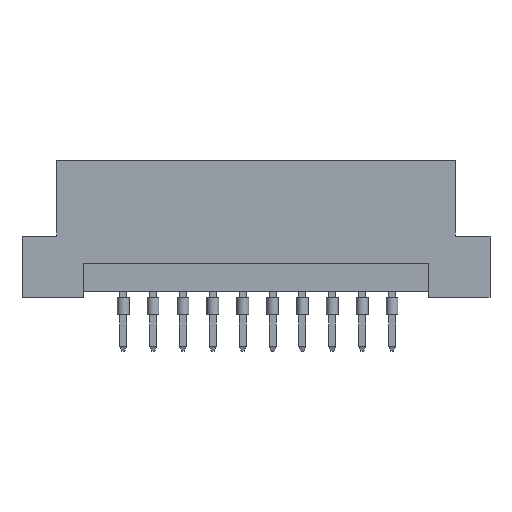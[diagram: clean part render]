
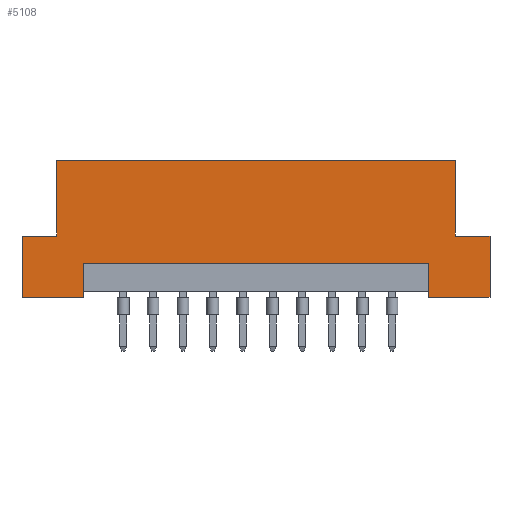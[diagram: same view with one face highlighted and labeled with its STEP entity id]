
A CAD part, front view. The second image highlights one B-rep face of the part: STEP entity #5108.
In plain terms, the highlighted planar face has unit normal (0, -1, 0).
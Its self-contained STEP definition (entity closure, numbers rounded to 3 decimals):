
#150 = CARTESIAN_POINT ( 'NONE',  ( 19.9, 0., 5.2 ) ) ;
#184 = DIRECTION ( 'NONE',  ( 0., 0., -1. ) ) ;
#199 = VECTOR ( 'NONE', #1365, 1000. ) ;
#215 = VERTEX_POINT ( 'NONE', #4006 ) ;
#225 = DIRECTION ( 'NONE',  ( 0., 0., 1. ) ) ;
#230 = LINE ( 'NONE', #5498, #4510 ) ;
#260 = DIRECTION ( 'NONE',  ( -1., 0., 0. ) ) ;
#274 = ORIENTED_EDGE ( 'NONE', *, *, #7486, .F. ) ;
#414 = VECTOR ( 'NONE', #1257, 1000. ) ;
#516 = ORIENTED_EDGE ( 'NONE', *, *, #4968, .F. ) ;
#571 = CARTESIAN_POINT ( 'NONE',  ( -19.9, 0., 5.2 ) ) ;
#603 = AXIS2_PLACEMENT_3D ( 'NONE', #806, #7228, #225 ) ;
#608 = LINE ( 'NONE', #571, #4751 ) ;
#670 = CARTESIAN_POINT ( 'NONE',  ( 16.94, 0., 5.2 ) ) ;
#682 = DIRECTION ( 'NONE',  ( 0., 0., 1. ) ) ;
#714 = DIRECTION ( 'NONE',  ( 0., 0., 1. ) ) ;
#747 = VECTOR ( 'NONE', #714, 1000. ) ;
#806 = CARTESIAN_POINT ( 'NONE',  ( -19.9, 0., 11.6 ) ) ;
#909 = EDGE_CURVE ( 'NONE', #4019, #6713, #3039, .T. ) ;
#1257 = DIRECTION ( 'NONE',  ( 1., 0., 0. ) ) ;
#1327 = CARTESIAN_POINT ( 'NONE',  ( -19.9, 0., 0. ) ) ;
#1365 = DIRECTION ( 'NONE',  ( 1., 0., 0. ) ) ;
#1489 = DIRECTION ( 'NONE',  ( 0., 0., -1. ) ) ;
#1496 = VERTEX_POINT ( 'NONE', #6316 ) ;
#1533 = CARTESIAN_POINT ( 'NONE',  ( 19.9, 0., 0. ) ) ;
#1563 = EDGE_CURVE ( 'NONE', #215, #4696, #6860, .T. ) ;
#1729 = CARTESIAN_POINT ( 'NONE',  ( -19.9, 0., 5.2 ) ) ;
#1744 = ORIENTED_EDGE ( 'NONE', *, *, #5093, .T. ) ;
#1761 = VERTEX_POINT ( 'NONE', #5969 ) ;
#1875 = CARTESIAN_POINT ( 'NONE',  ( 19.9, 0., 0. ) ) ;
#1886 = VECTOR ( 'NONE', #2543, 1000. ) ;
#1890 = VECTOR ( 'NONE', #5689, 1000. ) ;
#2126 = ORIENTED_EDGE ( 'NONE', *, *, #2799, .F. ) ;
#2294 = DIRECTION ( 'NONE',  ( 1., 0., 0. ) ) ;
#2312 = CARTESIAN_POINT ( 'NONE',  ( -16.94, 0., 11.6 ) ) ;
#2412 = VECTOR ( 'NONE', #6301, 1000. ) ;
#2446 = EDGE_CURVE ( 'NONE', #6695, #6727, #2455, .T. ) ;
#2455 = LINE ( 'NONE', #3116, #1886 ) ;
#2543 = DIRECTION ( 'NONE',  ( -1., 0., 0. ) ) ;
#2573 = CARTESIAN_POINT ( 'NONE',  ( -19.9, 0., 11.6 ) ) ;
#2679 = VERTEX_POINT ( 'NONE', #1729 ) ;
#2797 = LINE ( 'NONE', #7532, #2412 ) ;
#2799 = EDGE_CURVE ( 'NONE', #1496, #5699, #4226, .T. ) ;
#2817 = EDGE_CURVE ( 'NONE', #5699, #2679, #5487, .T. ) ;
#2835 = EDGE_CURVE ( 'NONE', #4578, #5888, #6612, .T. ) ;
#3039 = LINE ( 'NONE', #150, #414 ) ;
#3116 = CARTESIAN_POINT ( 'NONE',  ( -19.9, 0., 0. ) ) ;
#3148 = EDGE_LOOP ( 'NONE', ( #5602, #1744, #7469, #274, #3656, #6616, #6815, #6595, #516, #4287, #2126, #4163 ) ) ;
#3265 = CARTESIAN_POINT ( 'NONE',  ( 19.9, 0., 5.2 ) ) ;
#3335 = EDGE_CURVE ( 'NONE', #4696, #1496, #230, .T. ) ;
#3339 = VECTOR ( 'NONE', #682, 1000. ) ;
#3656 = ORIENTED_EDGE ( 'NONE', *, *, #909, .F. ) ;
#3796 = CARTESIAN_POINT ( 'NONE',  ( 14.69, 0., 0.5 ) ) ;
#4006 = CARTESIAN_POINT ( 'NONE',  ( 14.69, 0., 2.9 ) ) ;
#4019 = VERTEX_POINT ( 'NONE', #670 ) ;
#4043 = CARTESIAN_POINT ( 'NONE',  ( 16.94, 0., 11.6 ) ) ;
#4163 = ORIENTED_EDGE ( 'NONE', *, *, #3335, .F. ) ;
#4226 = LINE ( 'NONE', #1327, #7528 ) ;
#4242 = EDGE_CURVE ( 'NONE', #4019, #5888, #6067, .T. ) ;
#4287 = ORIENTED_EDGE ( 'NONE', *, *, #2817, .F. ) ;
#4510 = VECTOR ( 'NONE', #1489, 1000. ) ;
#4578 = VERTEX_POINT ( 'NONE', #2312 ) ;
#4696 = VERTEX_POINT ( 'NONE', #4888 ) ;
#4751 = VECTOR ( 'NONE', #2294, 1000. ) ;
#4840 = CARTESIAN_POINT ( 'NONE',  ( -19.9, 0., 0. ) ) ;
#4841 = PLANE ( 'NONE',  #603 ) ;
#4842 = EDGE_CURVE ( 'NONE', #1761, #4578, #2797, .T. ) ;
#4888 = CARTESIAN_POINT ( 'NONE',  ( -14.69, 0., 2.9 ) ) ;
#4968 = EDGE_CURVE ( 'NONE', #2679, #1761, #608, .T. ) ;
#5093 = EDGE_CURVE ( 'NONE', #215, #6727, #6113, .T. ) ;
#5108 = ADVANCED_FACE ( 'NONE', ( #5993 ), #4841, .F. ) ;
#5487 = LINE ( 'NONE', #4840, #3339 ) ;
#5498 = CARTESIAN_POINT ( 'NONE',  ( -14.69, 0., 0.5 ) ) ;
#5504 = CARTESIAN_POINT ( 'NONE',  ( 14.69, 0., 0. ) ) ;
#5598 = VECTOR ( 'NONE', #184, 1000. ) ;
#5602 = ORIENTED_EDGE ( 'NONE', *, *, #1563, .F. ) ;
#5689 = DIRECTION ( 'NONE',  ( -1., 0., 0. ) ) ;
#5699 = VERTEX_POINT ( 'NONE', #6246 ) ;
#5727 = CARTESIAN_POINT ( 'NONE',  ( 14.69, 0., 2.9 ) ) ;
#5888 = VERTEX_POINT ( 'NONE', #4043 ) ;
#5969 = CARTESIAN_POINT ( 'NONE',  ( -16.94, 0., 5.2 ) ) ;
#5972 = LINE ( 'NONE', #1875, #6077 ) ;
#5983 = CARTESIAN_POINT ( 'NONE',  ( 16.94, 0., 5.2 ) ) ;
#5993 = FACE_OUTER_BOUND ( 'NONE', #3148, .T. ) ;
#6067 = LINE ( 'NONE', #5983, #747 ) ;
#6077 = VECTOR ( 'NONE', #7211, 1000. ) ;
#6113 = LINE ( 'NONE', #3796, #5598 ) ;
#6246 = CARTESIAN_POINT ( 'NONE',  ( -19.9, 0., 0. ) ) ;
#6301 = DIRECTION ( 'NONE',  ( 0., 0., 1. ) ) ;
#6316 = CARTESIAN_POINT ( 'NONE',  ( -14.69, 0., 0. ) ) ;
#6595 = ORIENTED_EDGE ( 'NONE', *, *, #4842, .F. ) ;
#6612 = LINE ( 'NONE', #2573, #199 ) ;
#6616 = ORIENTED_EDGE ( 'NONE', *, *, #4242, .T. ) ;
#6695 = VERTEX_POINT ( 'NONE', #1533 ) ;
#6713 = VERTEX_POINT ( 'NONE', #3265 ) ;
#6727 = VERTEX_POINT ( 'NONE', #5504 ) ;
#6815 = ORIENTED_EDGE ( 'NONE', *, *, #2835, .F. ) ;
#6860 = LINE ( 'NONE', #5727, #1890 ) ;
#7211 = DIRECTION ( 'NONE',  ( 0., 0., -1. ) ) ;
#7228 = DIRECTION ( 'NONE',  ( 0., 1., 0. ) ) ;
#7469 = ORIENTED_EDGE ( 'NONE', *, *, #2446, .F. ) ;
#7486 = EDGE_CURVE ( 'NONE', #6713, #6695, #5972, .T. ) ;
#7528 = VECTOR ( 'NONE', #260, 1000. ) ;
#7532 = CARTESIAN_POINT ( 'NONE',  ( -16.94, 0., 5.2 ) ) ;
